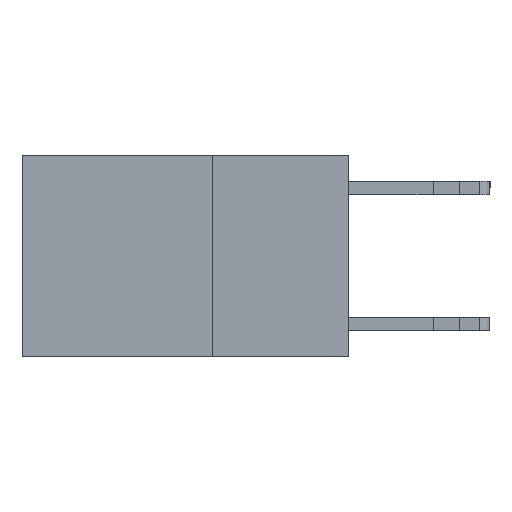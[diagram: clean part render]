
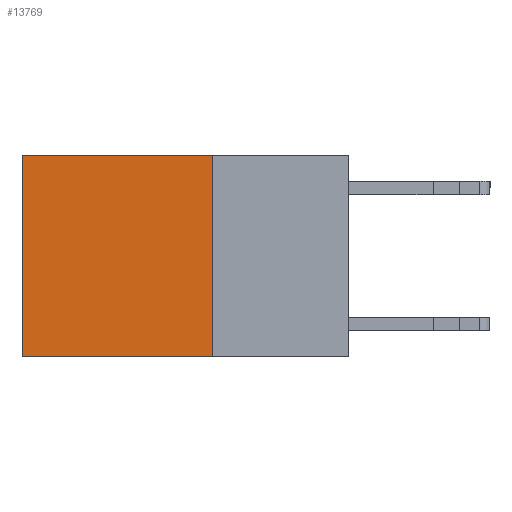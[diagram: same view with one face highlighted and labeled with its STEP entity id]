
A CAD part, left-side view. The second image highlights one B-rep face of the part: STEP entity #13769.
In plain terms, the highlighted planar face has unit normal (-1, 0, 0).
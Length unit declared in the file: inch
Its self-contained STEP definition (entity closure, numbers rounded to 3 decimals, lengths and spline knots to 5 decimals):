
#158 = EDGE_CURVE ( 'NONE', #11207, #17639, #17274, .T. ) ;
#2004 = EDGE_CURVE ( 'NONE', #7287, #2578, #18401, .T. ) ;
#2245 = CARTESIAN_POINT ( 'NONE',  ( 0.2625, 0.25, 0. ) ) ;
#2578 = VERTEX_POINT ( 'NONE', #7314 ) ;
#3528 = DIRECTION ( 'NONE',  ( 0., 0., -1. ) ) ;
#5395 = CARTESIAN_POINT ( 'NONE',  ( 0.2625, 0.25, 0. ) ) ;
#5399 = AXIS2_PLACEMENT_3D ( 'NONE', #5395, #15199, #11007 ) ;
#7112 = DIRECTION ( 'NONE',  ( 0., 0., -1. ) ) ;
#7128 = EDGE_CURVE ( 'NONE', #17639, #2578, #18362, .T. ) ;
#7287 = VERTEX_POINT ( 'NONE', #11971 ) ;
#7314 = CARTESIAN_POINT ( 'NONE',  ( 0.2625, 0.6, -0.37 ) ) ;
#7361 = DIRECTION ( 'NONE',  ( 0., 1., 0. ) ) ;
#9861 = CARTESIAN_POINT ( 'NONE',  ( 0.2625, 0.25, -0.37 ) ) ;
#10897 = VECTOR ( 'NONE', #7361, 39.37008 ) ;
#11007 = DIRECTION ( 'NONE',  ( 0., 0., -1. ) ) ;
#11171 = ORIENTED_EDGE ( 'NONE', *, *, #7128, .T. ) ;
#11207 = VERTEX_POINT ( 'NONE', #2245 ) ;
#11760 = EDGE_CURVE ( 'NONE', #11207, #7287, #12339, .T. ) ;
#11865 = FACE_OUTER_BOUND ( 'NONE', #18528, .T. ) ;
#11971 = CARTESIAN_POINT ( 'NONE',  ( 0.2625, 0.25, -0.37 ) ) ;
#12316 = PLANE ( 'NONE',  #5399 ) ;
#12339 = LINE ( 'NONE', #14957, #15196 ) ;
#13001 = ORIENTED_EDGE ( 'NONE', *, *, #11760, .F. ) ;
#13769 = ADVANCED_FACE ( 'NONE', ( #11865 ), #12316, .F. ) ;
#14360 = ORIENTED_EDGE ( 'NONE', *, *, #158, .T. ) ;
#14471 = CARTESIAN_POINT ( 'NONE',  ( 0.2625, 0.25, 0. ) ) ;
#14619 = VECTOR ( 'NONE', #7112, 39.37008 ) ;
#14957 = CARTESIAN_POINT ( 'NONE',  ( 0.2625, 0.25, 0. ) ) ;
#15196 = VECTOR ( 'NONE', #3528, 39.37008 ) ;
#15199 = DIRECTION ( 'NONE',  ( 1., 0., 0. ) ) ;
#17236 = CARTESIAN_POINT ( 'NONE',  ( 0.2625, 0.6, 0. ) ) ;
#17272 = VECTOR ( 'NONE', #17713, 39.37008 ) ;
#17274 = LINE ( 'NONE', #14471, #10897 ) ;
#17639 = VERTEX_POINT ( 'NONE', #17236 ) ;
#17713 = DIRECTION ( 'NONE',  ( 0., 1., 0. ) ) ;
#18353 = ORIENTED_EDGE ( 'NONE', *, *, #2004, .F. ) ;
#18362 = LINE ( 'NONE', #18554, #14619 ) ;
#18401 = LINE ( 'NONE', #9861, #17272 ) ;
#18528 = EDGE_LOOP ( 'NONE', ( #11171, #18353, #13001, #14360 ) ) ;
#18554 = CARTESIAN_POINT ( 'NONE',  ( 0.2625, 0.6, 0. ) ) ;
